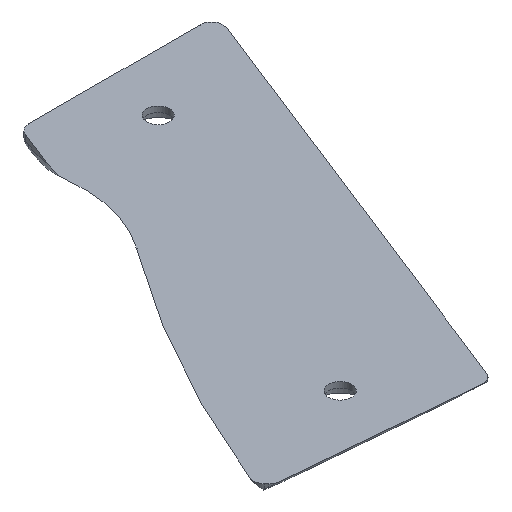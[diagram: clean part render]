
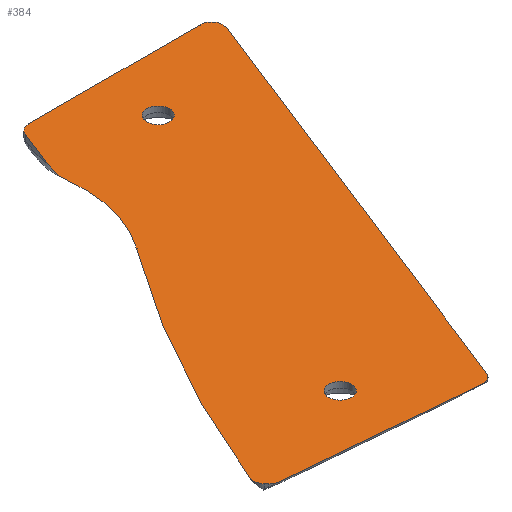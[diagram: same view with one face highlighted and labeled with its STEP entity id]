
A CAD part, isometric view. The second image highlights one B-rep face of the part: STEP entity #384.
In plain terms, the highlighted planar face has unit normal (0, 0, 1).
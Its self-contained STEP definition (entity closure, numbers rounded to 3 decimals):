
#17=FACE_BOUND('',#120,.T.);
#18=FACE_BOUND('',#121,.T.);
#23=PLANE('',#426);
#36=LINE('',#663,#57);
#37=LINE('',#667,#58);
#38=LINE('',#670,#59);
#39=LINE('',#678,#60);
#40=LINE('',#682,#61);
#57=VECTOR('',#491,10.);
#58=VECTOR('',#494,10.);
#59=VECTOR('',#497,10.);
#60=VECTOR('',#504,10.);
#61=VECTOR('',#507,10.);
#95=FACE_OUTER_BOUND('',#119,.T.);
#119=EDGE_LOOP('',(#283,#284,#285,#286,#287,#288,#289,#290,#291,#292,#293,
#294,#295));
#120=EDGE_LOOP('',(#296));
#121=EDGE_LOOP('',(#297));
#149=CIRCLE('',#427,2.);
#150=CIRCLE('',#428,2.);
#151=CIRCLE('',#429,22.992);
#152=CIRCLE('',#430,205.75);
#153=CIRCLE('',#431,2.);
#154=CIRCLE('',#432,2.);
#155=CIRCLE('',#433,2.);
#156=CIRCLE('',#434,2.);
#157=CIRCLE('',#435,2.);
#166=B_SPLINE_CURVE_WITH_KNOTS('',3,(#616,#617,#618,#619,#620,#621),
 .UNSPECIFIED.,.F.,.F.,(4,2,4),(0.,0.256,0.461),
 .UNSPECIFIED.);
#175=VERTEX_POINT('',#614);
#176=VERTEX_POINT('',#615);
#185=VERTEX_POINT('',#661);
#186=VERTEX_POINT('',#662);
#187=VERTEX_POINT('',#664);
#188=VERTEX_POINT('',#666);
#189=VERTEX_POINT('',#668);
#190=VERTEX_POINT('',#671);
#191=VERTEX_POINT('',#673);
#192=VERTEX_POINT('',#675);
#193=VERTEX_POINT('',#677);
#194=VERTEX_POINT('',#679);
#195=VERTEX_POINT('',#681);
#196=VERTEX_POINT('',#684);
#197=VERTEX_POINT('',#686);
#211=EDGE_CURVE('',#175,#176,#166,.T.);
#224=EDGE_CURVE('',#185,#186,#36,.T.);
#225=EDGE_CURVE('',#187,#185,#149,.T.);
#226=EDGE_CURVE('',#188,#187,#37,.T.);
#227=EDGE_CURVE('',#189,#188,#150,.T.);
#228=EDGE_CURVE('',#175,#189,#38,.T.);
#229=EDGE_CURVE('',#190,#176,#151,.T.);
#230=EDGE_CURVE('',#191,#190,#152,.T.);
#231=EDGE_CURVE('',#192,#191,#153,.T.);
#232=EDGE_CURVE('',#193,#192,#39,.T.);
#233=EDGE_CURVE('',#194,#193,#154,.T.);
#234=EDGE_CURVE('',#195,#194,#40,.T.);
#235=EDGE_CURVE('',#186,#195,#155,.T.);
#236=EDGE_CURVE('',#196,#196,#156,.T.);
#237=EDGE_CURVE('',#197,#197,#157,.T.);
#283=ORIENTED_EDGE('',*,*,#224,.F.);
#284=ORIENTED_EDGE('',*,*,#225,.F.);
#285=ORIENTED_EDGE('',*,*,#226,.F.);
#286=ORIENTED_EDGE('',*,*,#227,.F.);
#287=ORIENTED_EDGE('',*,*,#228,.F.);
#288=ORIENTED_EDGE('',*,*,#211,.T.);
#289=ORIENTED_EDGE('',*,*,#229,.F.);
#290=ORIENTED_EDGE('',*,*,#230,.F.);
#291=ORIENTED_EDGE('',*,*,#231,.F.);
#292=ORIENTED_EDGE('',*,*,#232,.F.);
#293=ORIENTED_EDGE('',*,*,#233,.F.);
#294=ORIENTED_EDGE('',*,*,#234,.F.);
#295=ORIENTED_EDGE('',*,*,#235,.F.);
#296=ORIENTED_EDGE('',*,*,#236,.F.);
#297=ORIENTED_EDGE('',*,*,#237,.F.);
#384=ADVANCED_FACE('',(#95,#17,#18),#23,.F.);
#426=AXIS2_PLACEMENT_3D('',#660,#489,#490);
#427=AXIS2_PLACEMENT_3D('',#665,#492,#493);
#428=AXIS2_PLACEMENT_3D('',#669,#495,#496);
#429=AXIS2_PLACEMENT_3D('',#672,#498,#499);
#430=AXIS2_PLACEMENT_3D('',#674,#500,#501);
#431=AXIS2_PLACEMENT_3D('',#676,#502,#503);
#432=AXIS2_PLACEMENT_3D('',#680,#505,#506);
#433=AXIS2_PLACEMENT_3D('',#683,#508,#509);
#434=AXIS2_PLACEMENT_3D('',#685,#510,#511);
#435=AXIS2_PLACEMENT_3D('',#687,#512,#513);
#489=DIRECTION('center_axis',(0.,0.,-1.));
#490=DIRECTION('ref_axis',(1.,0.,0.));
#491=DIRECTION('',(-0.367,-0.93,0.));
#492=DIRECTION('center_axis',(0.,0.,-1.));
#493=DIRECTION('ref_axis',(0.827,0.563,0.));
#494=DIRECTION('',(1.,0.,0.));
#495=DIRECTION('center_axis',(0.,0.,-1.));
#496=DIRECTION('ref_axis',(-0.563,0.827,0.));
#497=DIRECTION('',(0.367,0.93,0.));
#498=DIRECTION('center_axis',(0.,0.,1.));
#499=DIRECTION('ref_axis',(0.98,0.2,0.));
#500=DIRECTION('center_axis',(0.,0.,-1.));
#501=DIRECTION('ref_axis',(-0.93,0.367,0.));
#502=DIRECTION('center_axis',(0.,0.,-1.));
#503=DIRECTION('ref_axis',(-0.982,-0.191,0.));
#504=DIRECTION('',(-0.694,0.72,0.));
#505=DIRECTION('center_axis',(0.,0.,-1.));
#506=DIRECTION('ref_axis',(-0.432,-0.902,0.));
#507=DIRECTION('',(-0.996,0.089,0.));
#508=DIRECTION('center_axis',(0.,0.,-1.));
#509=DIRECTION('ref_axis',(0.525,-0.851,0.));
#510=DIRECTION('center_axis',(0.,0.,1.));
#511=DIRECTION('ref_axis',(-1.,0.,0.));
#512=DIRECTION('center_axis',(0.,0.,1.));
#513=DIRECTION('ref_axis',(-1.,0.,0.));
#614=CARTESIAN_POINT('',(72.113,-20.751,13.9));
#615=CARTESIAN_POINT('',(71.292,-24.879,13.9));
#616=CARTESIAN_POINT('Ctrl Pts',(72.113,-20.751,13.9));
#617=CARTESIAN_POINT('Ctrl Pts',(71.801,-21.544,13.9));
#618=CARTESIAN_POINT('Ctrl Pts',(71.518,-22.4,13.9));
#619=CARTESIAN_POINT('Ctrl Pts',(71.25,-23.906,13.9));
#620=CARTESIAN_POINT('Ctrl Pts',(71.237,-24.448,13.9));
#621=CARTESIAN_POINT('Ctrl Pts',(71.292,-24.879,13.9));
#660=CARTESIAN_POINT('Origin',(84.373,-48.148,13.9));
#661=CARTESIAN_POINT('',(108.4,-15.796,13.9));
#662=CARTESIAN_POINT('',(78.8,-90.939,13.9));
#663=CARTESIAN_POINT('',(101.337,-33.725,13.9));
#664=CARTESIAN_POINT('',(106.539,-13.063,13.9));
#665=CARTESIAN_POINT('Origin',(106.539,-15.063,13.9));
#666=CARTESIAN_POINT('',(76.503,-13.063,13.9));
#667=CARTESIAN_POINT('',(80.353,-13.063,13.9));
#668=CARTESIAN_POINT('',(74.642,-14.33,13.9));
#669=CARTESIAN_POINT('Origin',(76.503,-15.063,13.9));
#670=CARTESIAN_POINT('',(67.859,-31.55,13.9));
#671=CARTESIAN_POINT('',(67.093,-41.331,13.9));
#672=CARTESIAN_POINT('Origin',(48.489,-27.821,13.9));
#673=CARTESIAN_POINT('',(42.153,-86.164,13.9));
#674=CARTESIAN_POINT('Origin',(233.022,-162.989,13.9));
#675=CARTESIAN_POINT('',(42.568,-88.298,13.9));
#676=CARTESIAN_POINT('Origin',(44.008,-86.91,13.9));
#677=CARTESIAN_POINT('',(42.942,-88.686,13.9));
#678=CARTESIAN_POINT('',(42.819,-88.558,13.9));
#679=CARTESIAN_POINT('',(44.204,-89.29,13.9));
#680=CARTESIAN_POINT('Origin',(44.382,-87.298,13.9));
#681=CARTESIAN_POINT('',(76.762,-92.198,13.9));
#682=CARTESIAN_POINT('',(78.679,-92.369,13.9));
#683=CARTESIAN_POINT('Origin',(76.94,-90.206,13.9));
#684=CARTESIAN_POINT('',(91.132,-23.118,13.9));
#685=CARTESIAN_POINT('Origin',(89.132,-23.118,13.9));
#686=CARTESIAN_POINT('',(65.292,-80.791,13.9));
#687=CARTESIAN_POINT('Origin',(63.292,-80.791,13.9));
